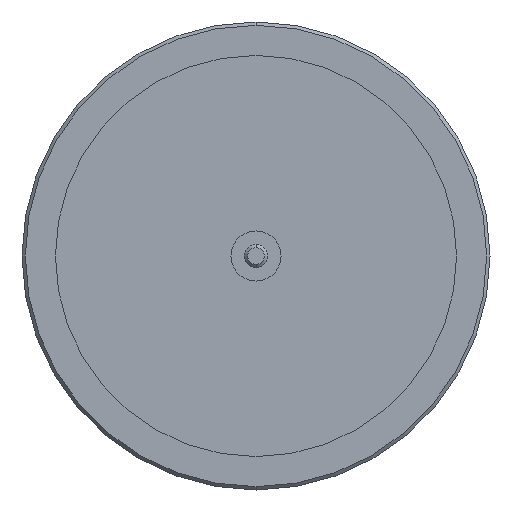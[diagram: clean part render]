
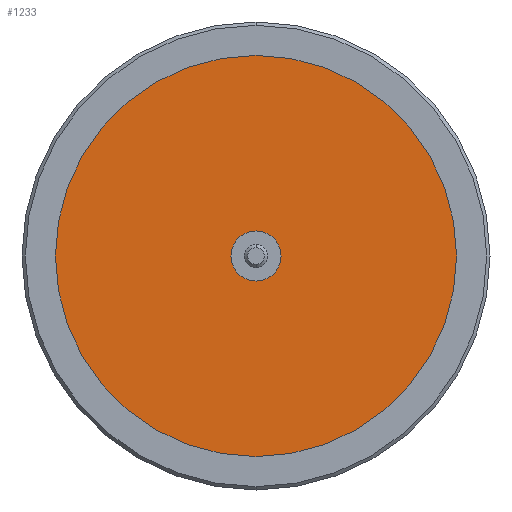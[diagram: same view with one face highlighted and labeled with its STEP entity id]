
A CAD part, front view. The second image highlights one B-rep face of the part: STEP entity #1233.
In plain terms, the highlighted planar face has unit normal (0, -1, 0).
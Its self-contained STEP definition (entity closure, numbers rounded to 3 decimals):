
#42 = CARTESIAN_POINT ( 'NONE',  ( 0., -2.1, 0.75 ) ) ;
#66 = VERTEX_POINT ( 'NONE', #1350 ) ;
#153 = CARTESIAN_POINT ( 'NONE',  ( 0., -2.1, 0. ) ) ;
#255 = DIRECTION ( 'NONE',  ( 0., 0., -1. ) ) ;
#262 = DIRECTION ( 'NONE',  ( 0., -1., 0. ) ) ;
#289 = DIRECTION ( 'NONE',  ( 0., -1., 0. ) ) ;
#305 = ORIENTED_EDGE ( 'NONE', *, *, #1224, .F. ) ;
#307 = EDGE_CURVE ( 'NONE', #1798, #66, #375, .T. ) ;
#375 = CIRCLE ( 'NONE', #1385, 6. ) ;
#407 = DIRECTION ( 'NONE',  ( 0., 0., -1. ) ) ;
#416 = EDGE_LOOP ( 'NONE', ( #1612, #1629 ) ) ;
#486 = VERTEX_POINT ( 'NONE', #42 ) ;
#517 = CIRCLE ( 'NONE', #974, 0.75 ) ;
#610 = CARTESIAN_POINT ( 'NONE',  ( 0., -2.1, 0. ) ) ;
#680 = AXIS2_PLACEMENT_3D ( 'NONE', #153, #262, #964 ) ;
#779 = ORIENTED_EDGE ( 'NONE', *, *, #1282, .F. ) ;
#872 = EDGE_CURVE ( 'NONE', #66, #1798, #1238, .T. ) ;
#950 = FACE_BOUND ( 'NONE', #1230, .T. ) ;
#964 = DIRECTION ( 'NONE',  ( 0., 0., -1. ) ) ;
#974 = AXIS2_PLACEMENT_3D ( 'NONE', #1210, #1244, #255 ) ;
#983 = DIRECTION ( 'NONE',  ( 0., -1., 0. ) ) ;
#987 = CARTESIAN_POINT ( 'NONE',  ( 0., -2.1, -6. ) ) ;
#1210 = CARTESIAN_POINT ( 'NONE',  ( 0., -2.1, 0. ) ) ;
#1224 = EDGE_CURVE ( 'NONE', #486, #1660, #517, .T. ) ;
#1230 = EDGE_LOOP ( 'NONE', ( #305, #779 ) ) ;
#1233 = ADVANCED_FACE ( 'NONE', ( #950, #1360 ), #1366, .T. ) ;
#1238 = CIRCLE ( 'NONE', #1712, 6. ) ;
#1244 = DIRECTION ( 'NONE',  ( 0., -1., 0. ) ) ;
#1255 = DIRECTION ( 'NONE',  ( 0., -1., 0. ) ) ;
#1282 = EDGE_CURVE ( 'NONE', #1660, #486, #1735, .T. ) ;
#1296 = DIRECTION ( 'NONE',  ( 0., 0., -1. ) ) ;
#1350 = CARTESIAN_POINT ( 'NONE',  ( 0., -2.1, 6. ) ) ;
#1360 = FACE_OUTER_BOUND ( 'NONE', #416, .T. ) ;
#1366 = PLANE ( 'NONE',  #680 ) ;
#1385 = AXIS2_PLACEMENT_3D ( 'NONE', #1544, #1255, #1296 ) ;
#1544 = CARTESIAN_POINT ( 'NONE',  ( 0., -2.1, 0. ) ) ;
#1567 = DIRECTION ( 'NONE',  ( 0., 0., -1. ) ) ;
#1612 = ORIENTED_EDGE ( 'NONE', *, *, #872, .T. ) ;
#1629 = ORIENTED_EDGE ( 'NONE', *, *, #307, .T. ) ;
#1639 = AXIS2_PLACEMENT_3D ( 'NONE', #1665, #289, #407 ) ;
#1656 = CARTESIAN_POINT ( 'NONE',  ( 0., -2.1, -0.75 ) ) ;
#1660 = VERTEX_POINT ( 'NONE', #1656 ) ;
#1665 = CARTESIAN_POINT ( 'NONE',  ( 0., -2.1, 0. ) ) ;
#1712 = AXIS2_PLACEMENT_3D ( 'NONE', #610, #983, #1567 ) ;
#1735 = CIRCLE ( 'NONE', #1639, 0.75 ) ;
#1798 = VERTEX_POINT ( 'NONE', #987 ) ;
